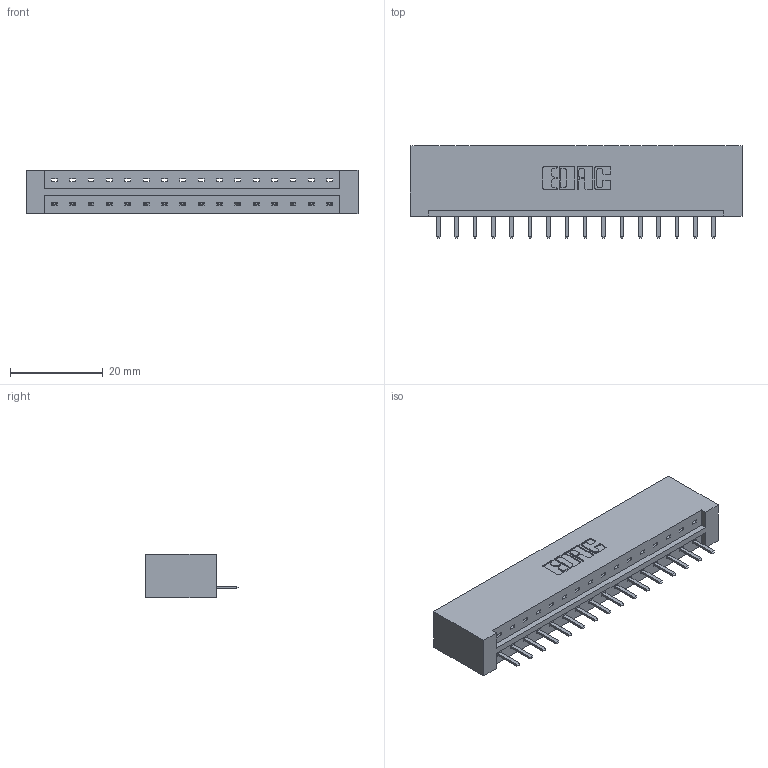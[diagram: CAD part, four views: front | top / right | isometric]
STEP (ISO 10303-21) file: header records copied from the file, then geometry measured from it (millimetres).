
FILE_DESCRIPTION (( 'STEP AP203' ), '1' );
FILE_NAME ('833-016-520-101.STEP', '2020-05-31T16:46:59', ( '' ), ( '' ), 'SwSTEP 2.0', 'SolidWorks 2020', '' );
FILE_SCHEMA (( 'CONFIG_CONTROL_DESIGN' ));
Length unit declared in the file: inch
Products named in the file (3): 833-016-520-101; 833 Part_Lugless; 345-292-001_345-293-120
Assembly tree (17 placements, depth 2):
  833-016-520-101
    833 Part_Lugless
    345-292-001_345-293-120  x16
Bounding box: 71.65 x 20.02 x 9.4 mm (x, y, z)
Volume: 7553.5 mm3; surface area: 7797.6 mm2
Topology: 17 solids, 17 shells, 1098 faces, 3231 edges, 2110 vertices
Faces by surface type: plane 770, cylinder 328
Entity records: 12981 total; most frequent: CARTESIAN_POINT 2262, ORIENTED_EDGE 2202, DIRECTION 1941, EDGE_CURVE 1101, VECTOR 977, LINE 977, VERTEX_POINT 730, AXIS2_PLACEMENT_3D 482
